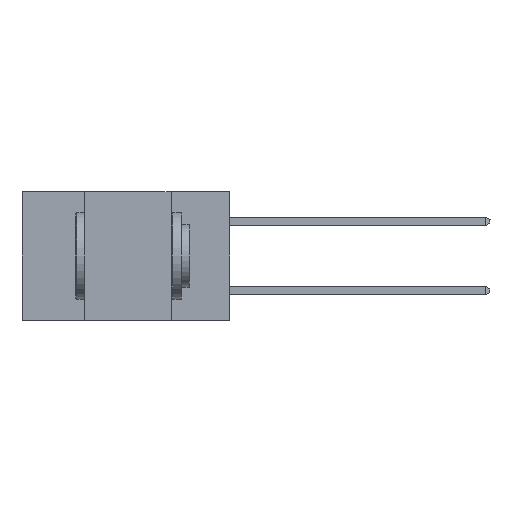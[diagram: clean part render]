
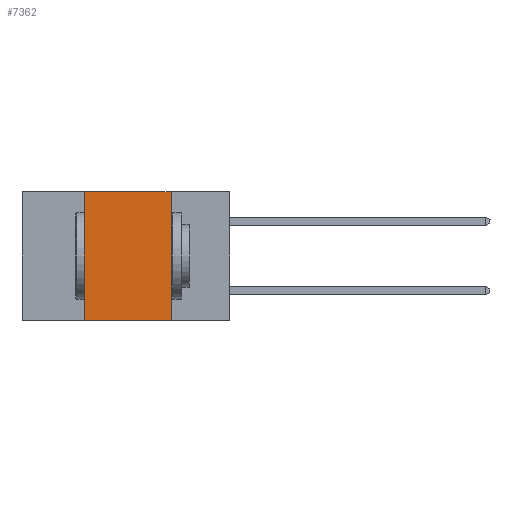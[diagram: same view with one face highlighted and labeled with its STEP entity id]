
A CAD part, left-side view. The second image highlights one B-rep face of the part: STEP entity #7362.
In plain terms, the highlighted planar face has unit normal (-1, 0, 0).
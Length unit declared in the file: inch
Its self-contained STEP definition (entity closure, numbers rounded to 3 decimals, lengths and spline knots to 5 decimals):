
#433 = VECTOR ( 'NONE', #8506, 39.37008 ) ;
#697 = VECTOR ( 'NONE', #8952, 39.37008 ) ;
#706 = LINE ( 'NONE', #9352, #433 ) ;
#1463 = LINE ( 'NONE', #9239, #10599 ) ;
#3053 = ORIENTED_EDGE ( 'NONE', *, *, #5593, .F. ) ;
#3191 = AXIS2_PLACEMENT_3D ( 'NONE', #6375, #6297, #12974 ) ;
#3968 = VERTEX_POINT ( 'NONE', #9664 ) ;
#4105 = VERTEX_POINT ( 'NONE', #9950 ) ;
#5015 = DIRECTION ( 'NONE',  ( 0., 0., 1. ) ) ;
#5271 = EDGE_CURVE ( 'NONE', #12787, #4105, #706, .T. ) ;
#5593 = EDGE_CURVE ( 'NONE', #3968, #12787, #1463, .T. ) ;
#6297 = DIRECTION ( 'NONE',  ( 1., 0., 0. ) ) ;
#6375 = CARTESIAN_POINT ( 'NONE',  ( 0., 0.6, 0. ) ) ;
#6467 = ORIENTED_EDGE ( 'NONE', *, *, #13113, .F. ) ;
#7114 = LINE ( 'NONE', #12357, #697 ) ;
#7242 = LINE ( 'NONE', #12857, #8456 ) ;
#7362 = ADVANCED_FACE ( 'NONE', ( #9679 ), #9831, .F. ) ;
#7708 = EDGE_LOOP ( 'NONE', ( #6467, #10012, #3053, #10141 ) ) ;
#7889 = EDGE_CURVE ( 'NONE', #3968, #13697, #7114, .T. ) ;
#8456 = VECTOR ( 'NONE', #9630, 39.37008 ) ;
#8506 = DIRECTION ( 'NONE',  ( 0., -1., 0. ) ) ;
#8952 = DIRECTION ( 'NONE',  ( 0., -1., 0. ) ) ;
#9239 = CARTESIAN_POINT ( 'NONE',  ( 0., 0.42, -0.37 ) ) ;
#9352 = CARTESIAN_POINT ( 'NONE',  ( 0., 0.6, 0. ) ) ;
#9630 = DIRECTION ( 'NONE',  ( 0., 0., -1. ) ) ;
#9645 = CARTESIAN_POINT ( 'NONE',  ( 0., 0.42, 0. ) ) ;
#9664 = CARTESIAN_POINT ( 'NONE',  ( 0., 0.42, -0.37 ) ) ;
#9679 = FACE_OUTER_BOUND ( 'NONE', #7708, .T. ) ;
#9753 = CARTESIAN_POINT ( 'NONE',  ( 0., 0.17, -0.37 ) ) ;
#9831 = PLANE ( 'NONE',  #3191 ) ;
#9950 = CARTESIAN_POINT ( 'NONE',  ( 0., 0.17, 0. ) ) ;
#10012 = ORIENTED_EDGE ( 'NONE', *, *, #5271, .F. ) ;
#10141 = ORIENTED_EDGE ( 'NONE', *, *, #7889, .T. ) ;
#10599 = VECTOR ( 'NONE', #5015, 39.37008 ) ;
#12357 = CARTESIAN_POINT ( 'NONE',  ( 0., 0.6, -0.37 ) ) ;
#12787 = VERTEX_POINT ( 'NONE', #9645 ) ;
#12857 = CARTESIAN_POINT ( 'NONE',  ( 0., 0.17, -0.37 ) ) ;
#12974 = DIRECTION ( 'NONE',  ( 0., 0., -1. ) ) ;
#13113 = EDGE_CURVE ( 'NONE', #4105, #13697, #7242, .T. ) ;
#13697 = VERTEX_POINT ( 'NONE', #9753 ) ;
